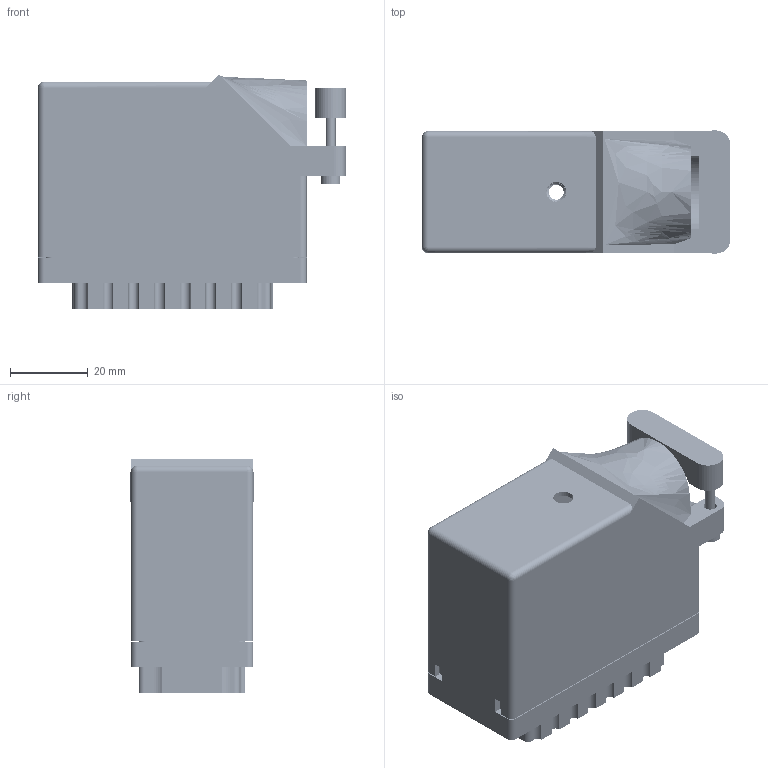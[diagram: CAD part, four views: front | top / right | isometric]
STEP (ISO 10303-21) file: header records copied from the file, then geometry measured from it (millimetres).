
FILE_DESCRIPTION (( 'STEP AP203' ), '1' );
FILE_NAME ('516-090-500-426.STEP', '2020-03-06T17:44:36', ( '' ), ( '' ), 'SwSTEP 2.0', 'SolidWorks 2016', '' );
FILE_SCHEMA (( 'CONFIG_CONTROL_DESIGN' ));
Length unit declared in the file: inch
Products named in the file (5): 516-252-095-100; 516 Part Receptacle_090; 516-230-001_Plastic - 090 Side Entry; 516-090-500-426; 516-292-001_500 Contact
Assembly tree (93 placements, depth 2):
  516-090-500-426
    516 Part Receptacle_090
    516-292-001_500 Contact  x90
    516-230-001_Plastic - 090 Side Entry
    516-252-095-100
Bounding box: 79.2 x 31.75 x 60.37 mm (x, y, z)
Volume: 40650.7 mm3; surface area: 68469.8 mm2
Topology: 93 solids, 93 shells, 8886 faces, 25835 edges, 17157 vertices
Faces by surface type: plane 5293, cylinder 3030, bspline 549, cone 12, sphere 2
Entity records: 76659 total; most frequent: CARTESIAN_POINT 15024, ORIENTED_EDGE 12506, DIRECTION 12169, EDGE_CURVE 6253, LINE 4571, VECTOR 4571, VERTEX_POINT 4163, AXIS2_PLACEMENT_3D 3799
